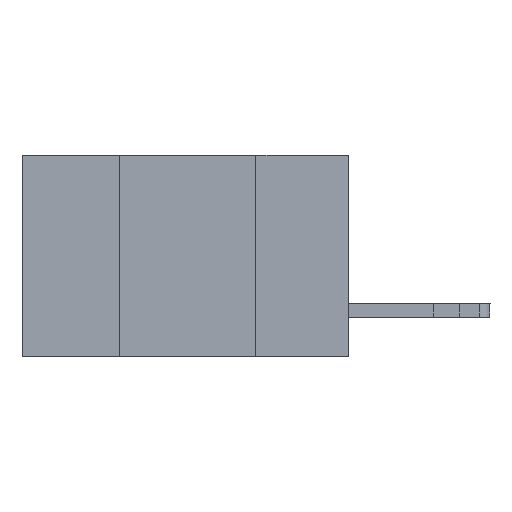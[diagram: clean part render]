
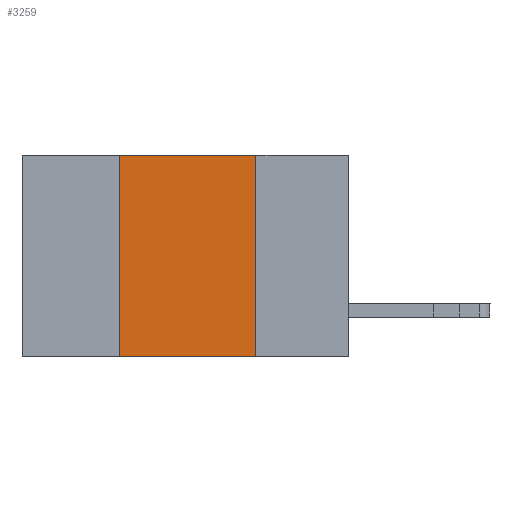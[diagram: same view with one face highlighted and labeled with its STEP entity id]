
A CAD part, left-side view. The second image highlights one B-rep face of the part: STEP entity #3259.
In plain terms, the highlighted planar face has unit normal (-1, 0, 0).
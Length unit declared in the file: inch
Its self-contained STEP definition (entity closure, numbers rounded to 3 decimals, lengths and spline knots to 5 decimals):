
#205 = CARTESIAN_POINT ( 'NONE',  ( 0., 0.42, -0.37 ) ) ;
#316 = EDGE_CURVE ( 'NONE', #6418, #7839, #13614, .T. ) ;
#1326 = CARTESIAN_POINT ( 'NONE',  ( 0., 0.6, 0. ) ) ;
#1464 = CARTESIAN_POINT ( 'NONE',  ( 0., 0.42, 0. ) ) ;
#1945 = CARTESIAN_POINT ( 'NONE',  ( 0., 0.6, 0. ) ) ;
#2404 = CARTESIAN_POINT ( 'NONE',  ( 0., 0.17, -0.37 ) ) ;
#3259 = ADVANCED_FACE ( 'NONE', ( #3975 ), #9936, .F. ) ;
#3290 = LINE ( 'NONE', #13722, #14600 ) ;
#3725 = VERTEX_POINT ( 'NONE', #12691 ) ;
#3975 = FACE_OUTER_BOUND ( 'NONE', #10352, .T. ) ;
#4178 = ORIENTED_EDGE ( 'NONE', *, *, #5792, .F. ) ;
#4646 = DIRECTION ( 'NONE',  ( 0., 0., -1. ) ) ;
#4690 = ORIENTED_EDGE ( 'NONE', *, *, #316, .F. ) ;
#5182 = DIRECTION ( 'NONE',  ( 0., -1., 0. ) ) ;
#5510 = VECTOR ( 'NONE', #13663, 39.37008 ) ;
#5792 = EDGE_CURVE ( 'NONE', #7839, #3725, #7259, .T. ) ;
#5863 = VECTOR ( 'NONE', #5182, 39.37008 ) ;
#6418 = VERTEX_POINT ( 'NONE', #205 ) ;
#7259 = LINE ( 'NONE', #1326, #5510 ) ;
#7633 = DIRECTION ( 'NONE',  ( 0., 0., -1. ) ) ;
#7839 = VERTEX_POINT ( 'NONE', #11897 ) ;
#8476 = AXIS2_PLACEMENT_3D ( 'NONE', #1945, #12241, #7633 ) ;
#9936 = PLANE ( 'NONE',  #8476 ) ;
#9994 = ORIENTED_EDGE ( 'NONE', *, *, #12179, .T. ) ;
#10352 = EDGE_LOOP ( 'NONE', ( #12287, #4178, #4690, #9994 ) ) ;
#10733 = CARTESIAN_POINT ( 'NONE',  ( 0., 0.6, -0.37 ) ) ;
#11169 = VERTEX_POINT ( 'NONE', #2404 ) ;
#11269 = LINE ( 'NONE', #10733, #5863 ) ;
#11479 = VECTOR ( 'NONE', #11567, 39.37008 ) ;
#11567 = DIRECTION ( 'NONE',  ( 0., 0., 1. ) ) ;
#11897 = CARTESIAN_POINT ( 'NONE',  ( 0., 0.42, 0. ) ) ;
#12179 = EDGE_CURVE ( 'NONE', #6418, #11169, #11269, .T. ) ;
#12241 = DIRECTION ( 'NONE',  ( 1., 0., 0. ) ) ;
#12287 = ORIENTED_EDGE ( 'NONE', *, *, #14132, .F. ) ;
#12691 = CARTESIAN_POINT ( 'NONE',  ( 0., 0.17, 0. ) ) ;
#13614 = LINE ( 'NONE', #1464, #11479 ) ;
#13663 = DIRECTION ( 'NONE',  ( 0., -1., 0. ) ) ;
#13722 = CARTESIAN_POINT ( 'NONE',  ( 0., 0.17, 0. ) ) ;
#14132 = EDGE_CURVE ( 'NONE', #3725, #11169, #3290, .T. ) ;
#14600 = VECTOR ( 'NONE', #4646, 39.37008 ) ;
